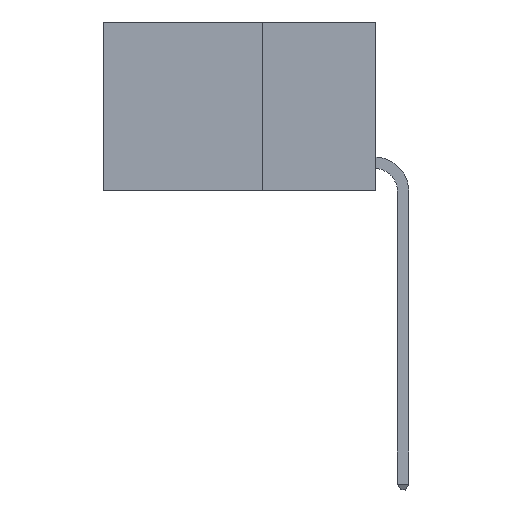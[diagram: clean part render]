
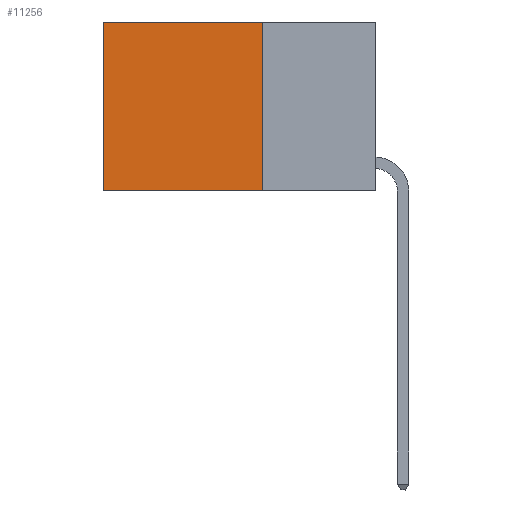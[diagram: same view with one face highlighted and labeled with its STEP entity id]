
A CAD part, left-side view. The second image highlights one B-rep face of the part: STEP entity #11256.
In plain terms, the highlighted planar face has unit normal (-1, 0, 0).
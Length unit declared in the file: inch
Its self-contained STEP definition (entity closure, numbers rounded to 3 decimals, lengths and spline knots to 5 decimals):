
#2074 = LINE ( 'NONE', #21144, #11214 ) ;
#2285 = VERTEX_POINT ( 'NONE', #15552 ) ;
#2580 = EDGE_LOOP ( 'NONE', ( #8840, #22360, #4597, #13967 ) ) ;
#2785 = DIRECTION ( 'NONE',  ( 0., 1., 0. ) ) ;
#4597 = ORIENTED_EDGE ( 'NONE', *, *, #11498, .F. ) ;
#5481 = EDGE_CURVE ( 'NONE', #7471, #23439, #12605, .T. ) ;
#6023 = EDGE_CURVE ( 'NONE', #22276, #23439, #15429, .T. ) ;
#6804 = CARTESIAN_POINT ( 'NONE',  ( 0.2625, 0.6, 0. ) ) ;
#7471 = VERTEX_POINT ( 'NONE', #12208 ) ;
#7797 = VECTOR ( 'NONE', #2785, 39.37008 ) ;
#7849 = CARTESIAN_POINT ( 'NONE',  ( 0.2625, 0.6, 0. ) ) ;
#8840 = ORIENTED_EDGE ( 'NONE', *, *, #6023, .T. ) ;
#9585 = AXIS2_PLACEMENT_3D ( 'NONE', #9793, #22327, #11578 ) ;
#9757 = DIRECTION ( 'NONE',  ( 0., 0., -1. ) ) ;
#9793 = CARTESIAN_POINT ( 'NONE',  ( 0.2625, 0.25, 0. ) ) ;
#10185 = CARTESIAN_POINT ( 'NONE',  ( 0.2625, 0.6, -0.37 ) ) ;
#11214 = VECTOR ( 'NONE', #22944, 39.37008 ) ;
#11256 = ADVANCED_FACE ( 'NONE', ( #21054 ), #20527, .F. ) ;
#11498 = EDGE_CURVE ( 'NONE', #2285, #7471, #2074, .T. ) ;
#11578 = DIRECTION ( 'NONE',  ( 0., 0., -1. ) ) ;
#12208 = CARTESIAN_POINT ( 'NONE',  ( 0.2625, 0.25, -0.37 ) ) ;
#12372 = CARTESIAN_POINT ( 'NONE',  ( 0.2625, 0.25, 0. ) ) ;
#12605 = LINE ( 'NONE', #22621, #7797 ) ;
#13443 = EDGE_CURVE ( 'NONE', #2285, #22276, #16203, .T. ) ;
#13967 = ORIENTED_EDGE ( 'NONE', *, *, #13443, .T. ) ;
#15429 = LINE ( 'NONE', #7849, #19618 ) ;
#15552 = CARTESIAN_POINT ( 'NONE',  ( 0.2625, 0.25, 0. ) ) ;
#16203 = LINE ( 'NONE', #12372, #20375 ) ;
#19618 = VECTOR ( 'NONE', #9757, 39.37008 ) ;
#20375 = VECTOR ( 'NONE', #21312, 39.37008 ) ;
#20527 = PLANE ( 'NONE',  #9585 ) ;
#21054 = FACE_OUTER_BOUND ( 'NONE', #2580, .T. ) ;
#21144 = CARTESIAN_POINT ( 'NONE',  ( 0.2625, 0.25, 0. ) ) ;
#21312 = DIRECTION ( 'NONE',  ( 0., 1., 0. ) ) ;
#22276 = VERTEX_POINT ( 'NONE', #6804 ) ;
#22327 = DIRECTION ( 'NONE',  ( 1., 0., 0. ) ) ;
#22360 = ORIENTED_EDGE ( 'NONE', *, *, #5481, .F. ) ;
#22621 = CARTESIAN_POINT ( 'NONE',  ( 0.2625, 0.25, -0.37 ) ) ;
#22944 = DIRECTION ( 'NONE',  ( 0., 0., -1. ) ) ;
#23439 = VERTEX_POINT ( 'NONE', #10185 ) ;
